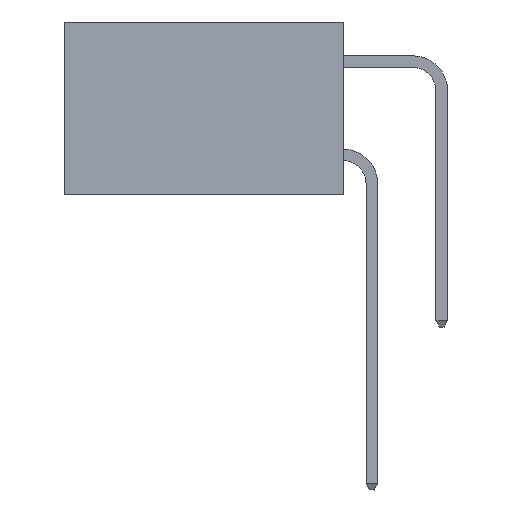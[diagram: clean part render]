
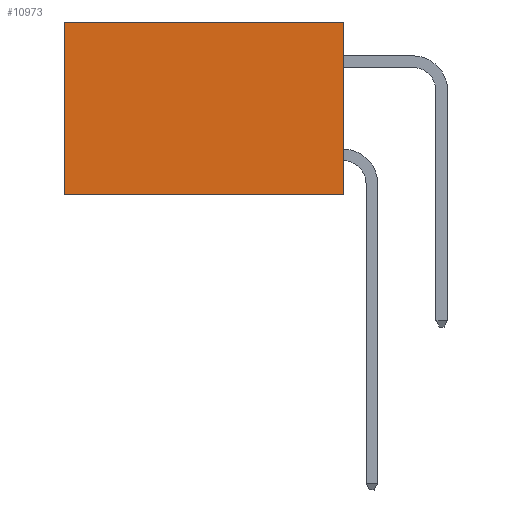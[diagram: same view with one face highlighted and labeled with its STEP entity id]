
A CAD part, left-side view. The second image highlights one B-rep face of the part: STEP entity #10973.
In plain terms, the highlighted planar face has unit normal (-1, 0, 0).
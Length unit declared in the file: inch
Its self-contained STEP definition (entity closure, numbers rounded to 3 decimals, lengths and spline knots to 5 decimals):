
#1036 = VECTOR ( 'NONE', #7483, 39.37008 ) ;
#1315 = FACE_OUTER_BOUND ( 'NONE', #2757, .T. ) ;
#1452 = VECTOR ( 'NONE', #7770, 39.37008 ) ;
#1975 = ORIENTED_EDGE ( 'NONE', *, *, #11179, .F. ) ;
#2319 = CARTESIAN_POINT ( 'NONE',  ( 0.298, 0., -0.37 ) ) ;
#2757 = EDGE_LOOP ( 'NONE', ( #12353, #1975, #10836, #10796 ) ) ;
#3540 = PLANE ( 'NONE',  #18193 ) ;
#5470 = CARTESIAN_POINT ( 'NONE',  ( 0.298, 0.6, -0.37 ) ) ;
#6034 = LINE ( 'NONE', #16226, #1452 ) ;
#6629 = DIRECTION ( 'NONE',  ( 0., 0., -1. ) ) ;
#7483 = DIRECTION ( 'NONE',  ( 0., 1., 0. ) ) ;
#7770 = DIRECTION ( 'NONE',  ( 0., 1., 0. ) ) ;
#7884 = EDGE_CURVE ( 'NONE', #9941, #12138, #6034, .T. ) ;
#8658 = DIRECTION ( 'NONE',  ( 0., 0., -1. ) ) ;
#9015 = CARTESIAN_POINT ( 'NONE',  ( 0.298, 0.6, 0. ) ) ;
#9621 = EDGE_CURVE ( 'NONE', #12138, #14333, #11534, .T. ) ;
#9941 = VERTEX_POINT ( 'NONE', #11625 ) ;
#10101 = LINE ( 'NONE', #2319, #1036 ) ;
#10796 = ORIENTED_EDGE ( 'NONE', *, *, #7884, .T. ) ;
#10836 = ORIENTED_EDGE ( 'NONE', *, *, #12212, .F. ) ;
#10973 = ADVANCED_FACE ( 'NONE', ( #1315 ), #3540, .F. ) ;
#11179 = EDGE_CURVE ( 'NONE', #19000, #14333, #10101, .T. ) ;
#11399 = VECTOR ( 'NONE', #6629, 39.37008 ) ;
#11529 = CARTESIAN_POINT ( 'NONE',  ( 0.298, 0.6, 0. ) ) ;
#11534 = LINE ( 'NONE', #9015, #19393 ) ;
#11625 = CARTESIAN_POINT ( 'NONE',  ( 0.298, 0., 0. ) ) ;
#12138 = VERTEX_POINT ( 'NONE', #11529 ) ;
#12212 = EDGE_CURVE ( 'NONE', #9941, #19000, #16456, .T. ) ;
#12353 = ORIENTED_EDGE ( 'NONE', *, *, #9621, .T. ) ;
#14333 = VERTEX_POINT ( 'NONE', #5470 ) ;
#14503 = CARTESIAN_POINT ( 'NONE',  ( 0.298, 0., -0.37 ) ) ;
#15081 = CARTESIAN_POINT ( 'NONE',  ( 0.298, 0., 0. ) ) ;
#16226 = CARTESIAN_POINT ( 'NONE',  ( 0.298, 0., 0. ) ) ;
#16456 = LINE ( 'NONE', #15081, #11399 ) ;
#17152 = CARTESIAN_POINT ( 'NONE',  ( 0.298, 0., 0. ) ) ;
#18193 = AXIS2_PLACEMENT_3D ( 'NONE', #17152, #18791, #8658 ) ;
#18791 = DIRECTION ( 'NONE',  ( 1., 0., 0. ) ) ;
#19000 = VERTEX_POINT ( 'NONE', #14503 ) ;
#19393 = VECTOR ( 'NONE', #20781, 39.37008 ) ;
#20781 = DIRECTION ( 'NONE',  ( 0., 0., -1. ) ) ;
